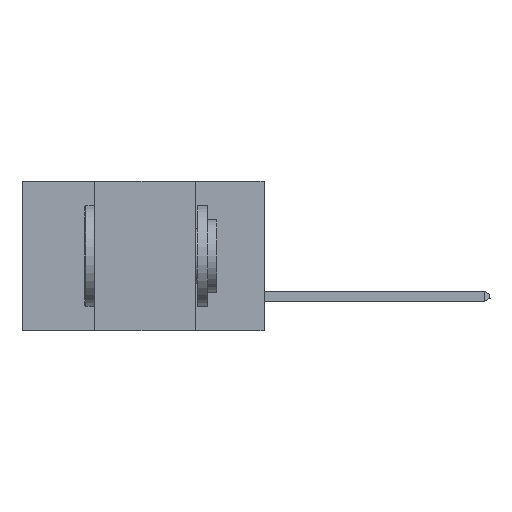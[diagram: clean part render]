
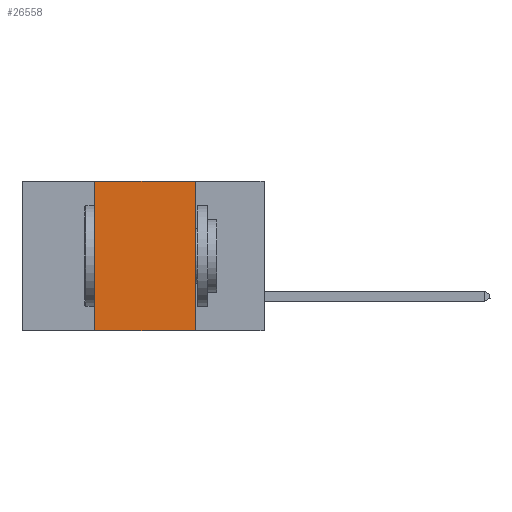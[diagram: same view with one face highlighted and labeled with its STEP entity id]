
A CAD part, left-side view. The second image highlights one B-rep face of the part: STEP entity #26558.
In plain terms, the highlighted planar face has unit normal (-1, 0, 0).
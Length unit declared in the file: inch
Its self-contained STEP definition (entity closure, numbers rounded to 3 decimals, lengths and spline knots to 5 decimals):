
#595 = VERTEX_POINT ( 'NONE', #18830 ) ;
#606 = DIRECTION ( 'NONE',  ( 0., -1., 0. ) ) ;
#829 = VECTOR ( 'NONE', #606, 39.37008 ) ;
#1286 = CARTESIAN_POINT ( 'NONE',  ( 0., 0.17, -0.37 ) ) ;
#1449 = VERTEX_POINT ( 'NONE', #18448 ) ;
#1505 = EDGE_LOOP ( 'NONE', ( #1654, #11595, #11650, #18641 ) ) ;
#1654 = ORIENTED_EDGE ( 'NONE', *, *, #8816, .F. ) ;
#2146 = LINE ( 'NONE', #13330, #829 ) ;
#3439 = DIRECTION ( 'NONE',  ( 0., 0., 1. ) ) ;
#3530 = CARTESIAN_POINT ( 'NONE',  ( 0., 0.42, 0. ) ) ;
#4149 = DIRECTION ( 'NONE',  ( 1., 0., 0. ) ) ;
#6843 = FACE_OUTER_BOUND ( 'NONE', #1505, .T. ) ;
#7032 = EDGE_CURVE ( 'NONE', #595, #26552, #2146, .T. ) ;
#8342 = PLANE ( 'NONE',  #19973 ) ;
#8816 = EDGE_CURVE ( 'NONE', #26552, #26137, #22132, .T. ) ;
#9535 = LINE ( 'NONE', #19879, #14484 ) ;
#10809 = DIRECTION ( 'NONE',  ( 0., 0., -1. ) ) ;
#11080 = CARTESIAN_POINT ( 'NONE',  ( 0., 0.17, 0. ) ) ;
#11438 = EDGE_CURVE ( 'NONE', #1449, #26137, #9535, .T. ) ;
#11595 = ORIENTED_EDGE ( 'NONE', *, *, #7032, .F. ) ;
#11650 = ORIENTED_EDGE ( 'NONE', *, *, #23952, .F. ) ;
#12604 = VECTOR ( 'NONE', #3439, 39.37008 ) ;
#13330 = CARTESIAN_POINT ( 'NONE',  ( 0., 0.6, 0. ) ) ;
#13943 = LINE ( 'NONE', #3530, #12604 ) ;
#14484 = VECTOR ( 'NONE', #26024, 39.37008 ) ;
#16694 = DIRECTION ( 'NONE',  ( 0., 0., -1. ) ) ;
#16894 = VECTOR ( 'NONE', #10809, 39.37008 ) ;
#18448 = CARTESIAN_POINT ( 'NONE',  ( 0., 0.42, -0.37 ) ) ;
#18641 = ORIENTED_EDGE ( 'NONE', *, *, #11438, .T. ) ;
#18719 = CARTESIAN_POINT ( 'NONE',  ( 0., 0.6, 0. ) ) ;
#18830 = CARTESIAN_POINT ( 'NONE',  ( 0., 0.42, 0. ) ) ;
#19835 = CARTESIAN_POINT ( 'NONE',  ( 0., 0.17, 0. ) ) ;
#19879 = CARTESIAN_POINT ( 'NONE',  ( 0., 0.6, -0.37 ) ) ;
#19973 = AXIS2_PLACEMENT_3D ( 'NONE', #18719, #4149, #16694 ) ;
#22132 = LINE ( 'NONE', #11080, #16894 ) ;
#23952 = EDGE_CURVE ( 'NONE', #1449, #595, #13943, .T. ) ;
#26024 = DIRECTION ( 'NONE',  ( 0., -1., 0. ) ) ;
#26137 = VERTEX_POINT ( 'NONE', #1286 ) ;
#26552 = VERTEX_POINT ( 'NONE', #19835 ) ;
#26558 = ADVANCED_FACE ( 'NONE', ( #6843 ), #8342, .F. ) ;
